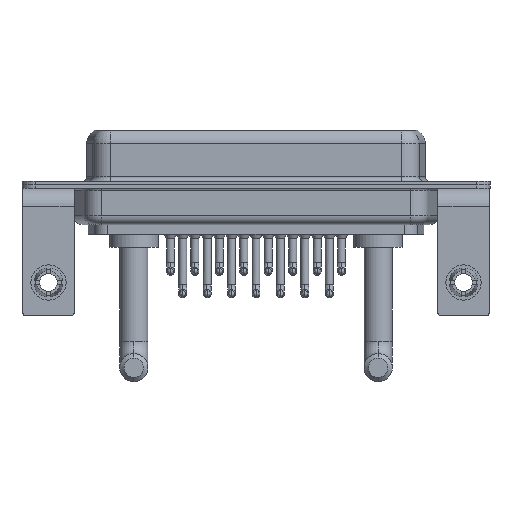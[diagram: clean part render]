
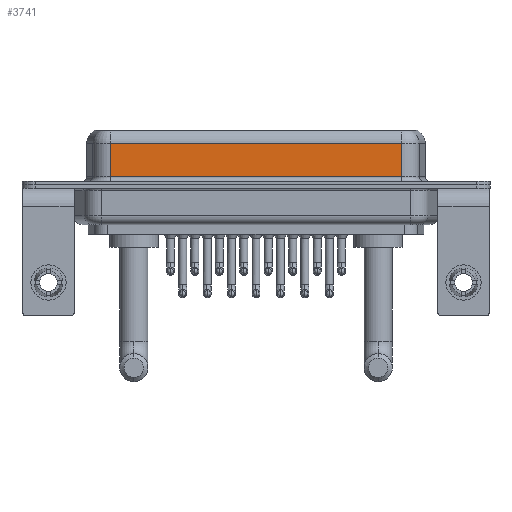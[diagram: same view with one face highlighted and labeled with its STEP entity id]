
A CAD part, front view. The second image highlights one B-rep face of the part: STEP entity #3741.
In plain terms, the highlighted planar face has unit normal (0, -1, 0).
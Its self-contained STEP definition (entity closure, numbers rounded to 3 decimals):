
#157 = EDGE_CURVE ( 'NONE', #2916, #14810, #22204, .T. ) ;
#296 = VERTEX_POINT ( 'NONE', #12997 ) ;
#506 = ORIENTED_EDGE ( 'NONE', *, *, #5000, .T. ) ;
#654 = ORIENTED_EDGE ( 'NONE', *, *, #157, .T. ) ;
#970 = ORIENTED_EDGE ( 'NONE', *, *, #3797, .F. ) ;
#2527 = CARTESIAN_POINT ( 'NONE',  ( 7.013, -3.95, 6.4 ) ) ;
#2759 = LINE ( 'NONE', #15319, #20320 ) ;
#2784 = AXIS2_PLACEMENT_3D ( 'NONE', #21532, #8957, #10814 ) ;
#2916 = VERTEX_POINT ( 'NONE', #6049 ) ;
#3741 = ADVANCED_FACE ( 'NONE', ( #14353 ), #16114, .F. ) ;
#3797 = EDGE_CURVE ( 'NONE', #16664, #14810, #9633, .T. ) ;
#4757 = DIRECTION ( 'NONE',  ( 0., 0., -1. ) ) ;
#5000 = EDGE_CURVE ( 'NONE', #296, #2916, #11572, .T. ) ;
#6049 = CARTESIAN_POINT ( 'NONE',  ( 7.013, -3.95, 0.9 ) ) ;
#6106 = CARTESIAN_POINT ( 'NONE',  ( 40.037, -3.95, 0.9 ) ) ;
#7319 = CARTESIAN_POINT ( 'NONE',  ( 40.037, -3.95, 4.65 ) ) ;
#7995 = DIRECTION ( 'NONE',  ( 0., 0., -1. ) ) ;
#8957 = DIRECTION ( 'NONE',  ( 0., 1., 0. ) ) ;
#9633 = LINE ( 'NONE', #22325, #10299 ) ;
#9917 = DIRECTION ( 'NONE',  ( -1., 0., 0. ) ) ;
#10299 = VECTOR ( 'NONE', #7995, 1000. ) ;
#10814 = DIRECTION ( 'NONE',  ( 0., 0., 1. ) ) ;
#11572 = LINE ( 'NONE', #2527, #16764 ) ;
#12087 = CARTESIAN_POINT ( 'NONE',  ( 40.037, -3.95, 0.9 ) ) ;
#12997 = CARTESIAN_POINT ( 'NONE',  ( 7.013, -3.95, 4.65 ) ) ;
#13117 = VECTOR ( 'NONE', #13271, 1000. ) ;
#13271 = DIRECTION ( 'NONE',  ( 1., 0., 0. ) ) ;
#14353 = FACE_OUTER_BOUND ( 'NONE', #18318, .T. ) ;
#14810 = VERTEX_POINT ( 'NONE', #12087 ) ;
#15319 = CARTESIAN_POINT ( 'NONE',  ( 40.037, -3.95, 4.65 ) ) ;
#16114 = PLANE ( 'NONE',  #2784 ) ;
#16577 = EDGE_CURVE ( 'NONE', #16664, #296, #2759, .T. ) ;
#16664 = VERTEX_POINT ( 'NONE', #7319 ) ;
#16764 = VECTOR ( 'NONE', #4757, 1000. ) ;
#18318 = EDGE_LOOP ( 'NONE', ( #970, #18560, #506, #654 ) ) ;
#18560 = ORIENTED_EDGE ( 'NONE', *, *, #16577, .T. ) ;
#20320 = VECTOR ( 'NONE', #9917, 1000. ) ;
#21532 = CARTESIAN_POINT ( 'NONE',  ( 40.037, -3.95, 6.4 ) ) ;
#22204 = LINE ( 'NONE', #6106, #13117 ) ;
#22325 = CARTESIAN_POINT ( 'NONE',  ( 40.037, -3.95, 6.4 ) ) ;
